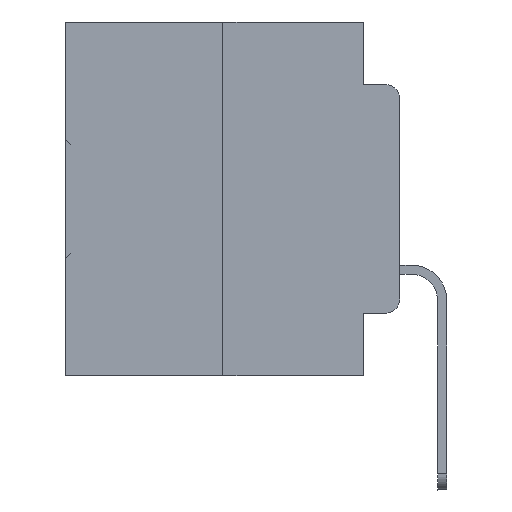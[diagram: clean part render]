
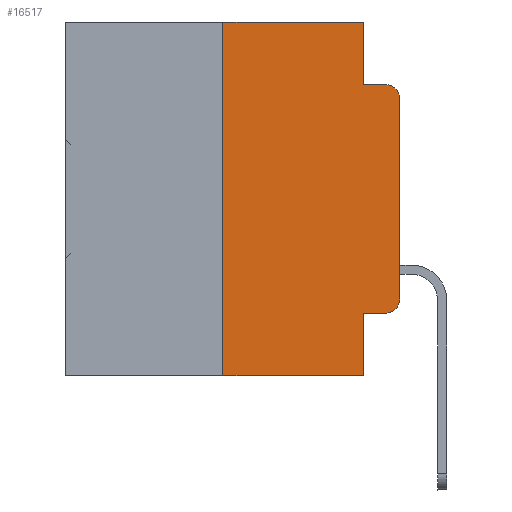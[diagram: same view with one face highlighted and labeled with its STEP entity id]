
A CAD part, left-side view. The second image highlights one B-rep face of the part: STEP entity #16517.
In plain terms, the highlighted planar face has unit normal (-1, 0, 0).
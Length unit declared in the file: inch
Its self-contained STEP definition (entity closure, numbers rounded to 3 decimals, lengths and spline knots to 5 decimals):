
#646 = ORIENTED_EDGE ( 'NONE', *, *, #13108, .F. ) ;
#1205 = CARTESIAN_POINT ( 'NONE',  ( 0., 0.473, 0. ) ) ;
#1326 = ORIENTED_EDGE ( 'NONE', *, *, #18339, .T. ) ;
#1359 = VECTOR ( 'NONE', #17496, 39.37008 ) ;
#1371 = ORIENTED_EDGE ( 'NONE', *, *, #20768, .F. ) ;
#1476 = CARTESIAN_POINT ( 'NONE',  ( 0., 0.473, 0. ) ) ;
#1579 = VECTOR ( 'NONE', #18644, 39.37008 ) ;
#1775 = CARTESIAN_POINT ( 'NONE',  ( 0., 0.02, -0.1085 ) ) ;
#1927 = ORIENTED_EDGE ( 'NONE', *, *, #3549, .F. ) ;
#2486 = DIRECTION ( 'NONE',  ( 0., 0., 1. ) ) ;
#2728 = DIRECTION ( 'NONE',  ( 0., 0., -1. ) ) ;
#2880 = CARTESIAN_POINT ( 'NONE',  ( 0., 0.473, -0.5 ) ) ;
#3394 = LINE ( 'NONE', #2880, #1579 ) ;
#3549 = EDGE_CURVE ( 'NONE', #29768, #6589, #15519, .T. ) ;
#4126 = CARTESIAN_POINT ( 'NONE',  ( 0., 0.25, 0. ) ) ;
#4478 = VECTOR ( 'NONE', #33092, 39.37008 ) ;
#4705 = LINE ( 'NONE', #20827, #1359 ) ;
#4870 = CARTESIAN_POINT ( 'NONE',  ( 0., 0.02, -0.3915 ) ) ;
#5377 = VERTEX_POINT ( 'NONE', #31485 ) ;
#5541 = AXIS2_PLACEMENT_3D ( 'NONE', #4870, #31501, #20985 ) ;
#6168 = CARTESIAN_POINT ( 'NONE',  ( 0., 0.051, -0.5 ) ) ;
#6482 = VERTEX_POINT ( 'NONE', #30874 ) ;
#6589 = VERTEX_POINT ( 'NONE', #14063 ) ;
#6753 = EDGE_CURVE ( 'NONE', #32672, #16527, #17577, .T. ) ;
#6765 = FACE_OUTER_BOUND ( 'NONE', #21461, .T. ) ;
#6903 = LINE ( 'NONE', #30551, #22841 ) ;
#6929 = DIRECTION ( 'NONE',  ( 1., 0., 0. ) ) ;
#8241 = CARTESIAN_POINT ( 'NONE',  ( 0., 0.051, 0. ) ) ;
#8268 = VERTEX_POINT ( 'NONE', #8300 ) ;
#8300 = CARTESIAN_POINT ( 'NONE',  ( 0., 0.25, -0.5 ) ) ;
#9961 = DIRECTION ( 'NONE',  ( 0., -1., 0. ) ) ;
#11758 = VECTOR ( 'NONE', #29698, 39.37008 ) ;
#12179 = DIRECTION ( 'NONE',  ( 0., 0., -1. ) ) ;
#12475 = VERTEX_POINT ( 'NONE', #4126 ) ;
#12771 = EDGE_CURVE ( 'NONE', #6482, #18479, #21621, .T. ) ;
#13005 = CARTESIAN_POINT ( 'NONE',  ( 0., 0., 0. ) ) ;
#13108 = EDGE_CURVE ( 'NONE', #6589, #16527, #33258, .T. ) ;
#14063 = CARTESIAN_POINT ( 'NONE',  ( 0., 0.051, -0.0885 ) ) ;
#15445 = LINE ( 'NONE', #13005, #22450 ) ;
#15519 = LINE ( 'NONE', #34619, #16835 ) ;
#16517 = ADVANCED_FACE ( 'NONE', ( #6765 ), #25499, .F. ) ;
#16527 = VERTEX_POINT ( 'NONE', #31962 ) ;
#16835 = VECTOR ( 'NONE', #2728, 39.37008 ) ;
#17313 = CARTESIAN_POINT ( 'NONE',  ( 0., 0.051, -0.0885 ) ) ;
#17329 = LINE ( 'NONE', #1205, #32473 ) ;
#17407 = DIRECTION ( 'NONE',  ( 0., 0., 1. ) ) ;
#17496 = DIRECTION ( 'NONE',  ( 0., -1., 0. ) ) ;
#17577 = CIRCLE ( 'NONE', #19268, 0.02 ) ;
#17862 = AXIS2_PLACEMENT_3D ( 'NONE', #1476, #6929, #12179 ) ;
#18065 = DIRECTION ( 'NONE',  ( -1., 0., 0. ) ) ;
#18339 = EDGE_CURVE ( 'NONE', #21686, #32672, #15445, .T. ) ;
#18479 = VERTEX_POINT ( 'NONE', #6168 ) ;
#18644 = DIRECTION ( 'NONE',  ( 0., -1., 0. ) ) ;
#18826 = CARTESIAN_POINT ( 'NONE',  ( 0., 0., -0.3915 ) ) ;
#19002 = CARTESIAN_POINT ( 'NONE',  ( 0., 0.051, 0. ) ) ;
#19268 = AXIS2_PLACEMENT_3D ( 'NONE', #1775, #18065, #23673 ) ;
#20768 = EDGE_CURVE ( 'NONE', #8268, #12475, #6903, .T. ) ;
#20827 = CARTESIAN_POINT ( 'NONE',  ( 0., 0.051, -0.4115 ) ) ;
#20985 = DIRECTION ( 'NONE',  ( 0., 0., -1. ) ) ;
#21461 = EDGE_LOOP ( 'NONE', ( #1326, #26038, #646, #1927, #30420, #1371, #26913, #33476, #24280, #31253 ) ) ;
#21621 = LINE ( 'NONE', #19002, #11758 ) ;
#21686 = VERTEX_POINT ( 'NONE', #18826 ) ;
#22450 = VECTOR ( 'NONE', #2486, 39.37008 ) ;
#22841 = VECTOR ( 'NONE', #17407, 39.37008 ) ;
#22961 = EDGE_CURVE ( 'NONE', #5377, #21686, #24582, .T. ) ;
#23673 = DIRECTION ( 'NONE',  ( 0., 0., -1. ) ) ;
#24119 = EDGE_CURVE ( 'NONE', #12475, #29768, #17329, .T. ) ;
#24280 = ORIENTED_EDGE ( 'NONE', *, *, #28783, .T. ) ;
#24582 = CIRCLE ( 'NONE', #5541, 0.02 ) ;
#25499 = PLANE ( 'NONE',  #17862 ) ;
#26038 = ORIENTED_EDGE ( 'NONE', *, *, #6753, .T. ) ;
#26527 = CARTESIAN_POINT ( 'NONE',  ( 0., 0., -0.1085 ) ) ;
#26913 = ORIENTED_EDGE ( 'NONE', *, *, #33981, .T. ) ;
#28783 = EDGE_CURVE ( 'NONE', #6482, #5377, #4705, .T. ) ;
#29698 = DIRECTION ( 'NONE',  ( 0., 0., -1. ) ) ;
#29768 = VERTEX_POINT ( 'NONE', #8241 ) ;
#30420 = ORIENTED_EDGE ( 'NONE', *, *, #24119, .F. ) ;
#30551 = CARTESIAN_POINT ( 'NONE',  ( 0., 0.25, 0. ) ) ;
#30874 = CARTESIAN_POINT ( 'NONE',  ( 0., 0.051, -0.4115 ) ) ;
#31253 = ORIENTED_EDGE ( 'NONE', *, *, #22961, .T. ) ;
#31485 = CARTESIAN_POINT ( 'NONE',  ( 0., 0.02, -0.4115 ) ) ;
#31501 = DIRECTION ( 'NONE',  ( -1., 0., 0. ) ) ;
#31962 = CARTESIAN_POINT ( 'NONE',  ( 0., 0.02, -0.0885 ) ) ;
#32473 = VECTOR ( 'NONE', #9961, 39.37008 ) ;
#32672 = VERTEX_POINT ( 'NONE', #26527 ) ;
#33092 = DIRECTION ( 'NONE',  ( 0., -1., 0. ) ) ;
#33258 = LINE ( 'NONE', #17313, #4478 ) ;
#33476 = ORIENTED_EDGE ( 'NONE', *, *, #12771, .F. ) ;
#33981 = EDGE_CURVE ( 'NONE', #8268, #18479, #3394, .T. ) ;
#34619 = CARTESIAN_POINT ( 'NONE',  ( 0., 0.051, 0. ) ) ;
